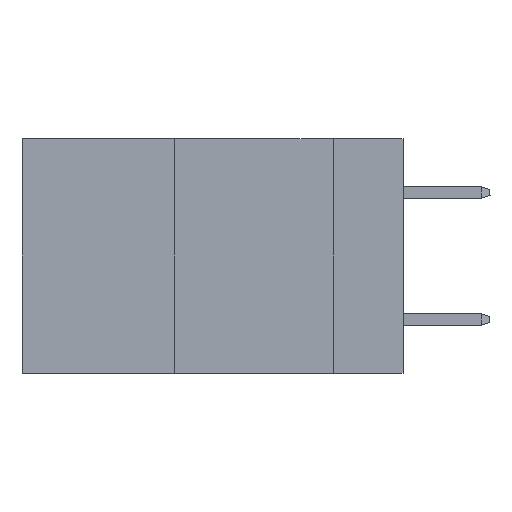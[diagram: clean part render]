
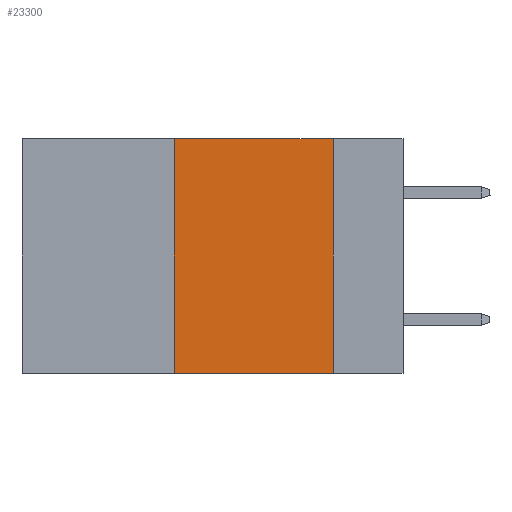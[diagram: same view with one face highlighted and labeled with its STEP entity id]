
A CAD part, left-side view. The second image highlights one B-rep face of the part: STEP entity #23300.
In plain terms, the highlighted planar face has unit normal (-1, 0, 0).
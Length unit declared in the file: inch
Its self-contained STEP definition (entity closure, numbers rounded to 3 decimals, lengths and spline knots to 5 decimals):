
#246 = CARTESIAN_POINT ( 'NONE',  ( 0., 0.36, 0. ) ) ;
#760 = CARTESIAN_POINT ( 'NONE',  ( 0., 0.11, 0. ) ) ;
#940 = EDGE_CURVE ( 'NONE', #33194, #22667, #18800, .T. ) ;
#1895 = DIRECTION ( 'NONE',  ( 0., -1., 0. ) ) ;
#4671 = DIRECTION ( 'NONE',  ( 0., 0., 1. ) ) ;
#5891 = DIRECTION ( 'NONE',  ( 0., -1., 0. ) ) ;
#6880 = DIRECTION ( 'NONE',  ( 0., 0., -1. ) ) ;
#7495 = EDGE_CURVE ( 'NONE', #11762, #21212, #14694, .T. ) ;
#7835 = VECTOR ( 'NONE', #5891, 39.37008 ) ;
#8770 = ORIENTED_EDGE ( 'NONE', *, *, #21010, .T. ) ;
#11762 = VERTEX_POINT ( 'NONE', #19760 ) ;
#12084 = FACE_OUTER_BOUND ( 'NONE', #33356, .T. ) ;
#12106 = VECTOR ( 'NONE', #6880, 39.37008 ) ;
#12647 = CARTESIAN_POINT ( 'NONE',  ( 0., 0.6, 0. ) ) ;
#14212 = CARTESIAN_POINT ( 'NONE',  ( 0., 0.6, -0.37 ) ) ;
#14227 = CARTESIAN_POINT ( 'NONE',  ( 0., 0.36, -0.37 ) ) ;
#14694 = LINE ( 'NONE', #760, #12106 ) ;
#14838 = DIRECTION ( 'NONE',  ( 0., 0., -1. ) ) ;
#15818 = CARTESIAN_POINT ( 'NONE',  ( 0., 0.11, -0.37 ) ) ;
#16160 = ORIENTED_EDGE ( 'NONE', *, *, #7495, .F. ) ;
#17618 = ORIENTED_EDGE ( 'NONE', *, *, #25180, .F. ) ;
#17788 = AXIS2_PLACEMENT_3D ( 'NONE', #12647, #23760, #14838 ) ;
#17938 = PLANE ( 'NONE',  #17788 ) ;
#18800 = LINE ( 'NONE', #35473, #21202 ) ;
#19760 = CARTESIAN_POINT ( 'NONE',  ( 0., 0.11, 0. ) ) ;
#21010 = EDGE_CURVE ( 'NONE', #33194, #21212, #30711, .T. ) ;
#21202 = VECTOR ( 'NONE', #4671, 39.37008 ) ;
#21212 = VERTEX_POINT ( 'NONE', #15818 ) ;
#21662 = LINE ( 'NONE', #27302, #25347 ) ;
#22667 = VERTEX_POINT ( 'NONE', #246 ) ;
#23300 = ADVANCED_FACE ( 'NONE', ( #12084 ), #17938, .F. ) ;
#23760 = DIRECTION ( 'NONE',  ( 1., 0., 0. ) ) ;
#25180 = EDGE_CURVE ( 'NONE', #22667, #11762, #21662, .T. ) ;
#25347 = VECTOR ( 'NONE', #1895, 39.37008 ) ;
#27302 = CARTESIAN_POINT ( 'NONE',  ( 0., 0.6, 0. ) ) ;
#30203 = ORIENTED_EDGE ( 'NONE', *, *, #940, .F. ) ;
#30711 = LINE ( 'NONE', #14212, #7835 ) ;
#33194 = VERTEX_POINT ( 'NONE', #14227 ) ;
#33356 = EDGE_LOOP ( 'NONE', ( #16160, #17618, #30203, #8770 ) ) ;
#35473 = CARTESIAN_POINT ( 'NONE',  ( 0., 0.36, 0. ) ) ;
